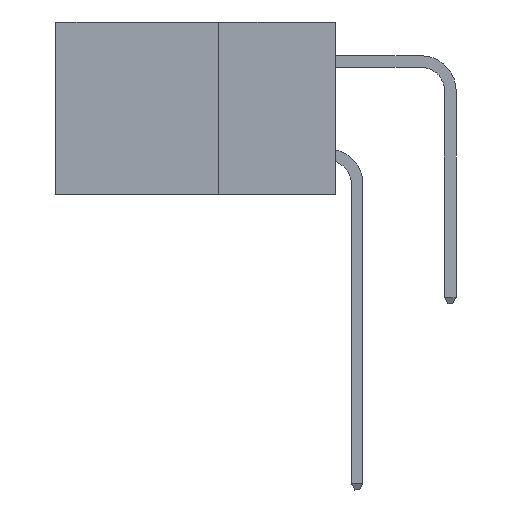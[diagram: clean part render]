
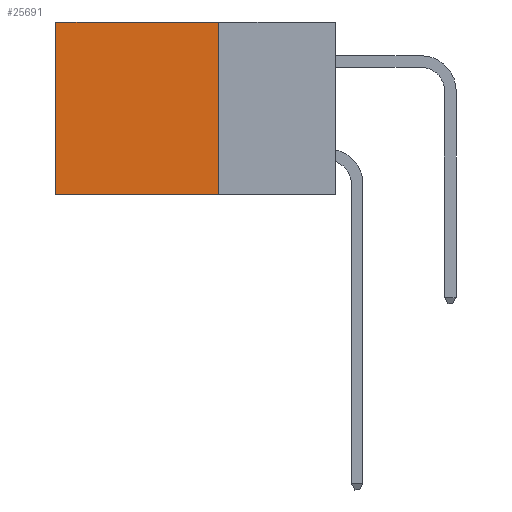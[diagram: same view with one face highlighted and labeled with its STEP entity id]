
A CAD part, left-side view. The second image highlights one B-rep face of the part: STEP entity #25691.
In plain terms, the highlighted planar face has unit normal (-1, 0, 0).
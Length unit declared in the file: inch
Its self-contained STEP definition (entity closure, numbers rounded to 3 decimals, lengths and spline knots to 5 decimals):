
#2548 = ORIENTED_EDGE ( 'NONE', *, *, #31524, .F. ) ;
#3533 = DIRECTION ( 'NONE',  ( 0., 0., -1. ) ) ;
#5704 = ORIENTED_EDGE ( 'NONE', *, *, #20865, .T. ) ;
#6212 = VECTOR ( 'NONE', #3533, 39.37008 ) ;
#8226 = EDGE_CURVE ( 'NONE', #35186, #17664, #32736, .T. ) ;
#8836 = DIRECTION ( 'NONE',  ( 0., 0., -1. ) ) ;
#9248 = FACE_OUTER_BOUND ( 'NONE', #13885, .T. ) ;
#9774 = DIRECTION ( 'NONE',  ( 0., 1., 0. ) ) ;
#9881 = VECTOR ( 'NONE', #24517, 39.37008 ) ;
#9988 = CARTESIAN_POINT ( 'NONE',  ( 0.2875, 0.25, -0.37 ) ) ;
#10068 = CARTESIAN_POINT ( 'NONE',  ( 0.2875, 0.25, 0. ) ) ;
#12613 = CARTESIAN_POINT ( 'NONE',  ( 0.2875, 0.6, 0. ) ) ;
#12982 = LINE ( 'NONE', #25811, #6212 ) ;
#13140 = LINE ( 'NONE', #9988, #15120 ) ;
#13885 = EDGE_LOOP ( 'NONE', ( #22132, #2548, #39092, #5704 ) ) ;
#14858 = LINE ( 'NONE', #27689, #9881 ) ;
#15120 = VECTOR ( 'NONE', #9774, 39.37008 ) ;
#16318 = CARTESIAN_POINT ( 'NONE',  ( 0.2875, 0.25, 0. ) ) ;
#17664 = VERTEX_POINT ( 'NONE', #25155 ) ;
#18876 = CARTESIAN_POINT ( 'NONE',  ( 0.2875, 0.6, -0.37 ) ) ;
#19999 = VECTOR ( 'NONE', #36100, 39.37008 ) ;
#20865 = EDGE_CURVE ( 'NONE', #35186, #25666, #14858, .T. ) ;
#22077 = PLANE ( 'NONE',  #39780 ) ;
#22132 = ORIENTED_EDGE ( 'NONE', *, *, #26334, .T. ) ;
#24517 = DIRECTION ( 'NONE',  ( 0., 1., 0. ) ) ;
#25155 = CARTESIAN_POINT ( 'NONE',  ( 0.2875, 0.25, -0.37 ) ) ;
#25666 = VERTEX_POINT ( 'NONE', #12613 ) ;
#25691 = ADVANCED_FACE ( 'NONE', ( #9248 ), #22077, .F. ) ;
#25811 = CARTESIAN_POINT ( 'NONE',  ( 0.2875, 0.6, 0. ) ) ;
#26334 = EDGE_CURVE ( 'NONE', #25666, #32419, #12982, .T. ) ;
#27689 = CARTESIAN_POINT ( 'NONE',  ( 0.2875, 0.25, 0. ) ) ;
#28607 = CARTESIAN_POINT ( 'NONE',  ( 0.2875, 0.25, 0. ) ) ;
#31349 = DIRECTION ( 'NONE',  ( 1., 0., 0. ) ) ;
#31524 = EDGE_CURVE ( 'NONE', #17664, #32419, #13140, .T. ) ;
#32419 = VERTEX_POINT ( 'NONE', #18876 ) ;
#32736 = LINE ( 'NONE', #16318, #19999 ) ;
#35186 = VERTEX_POINT ( 'NONE', #10068 ) ;
#36100 = DIRECTION ( 'NONE',  ( 0., 0., -1. ) ) ;
#39092 = ORIENTED_EDGE ( 'NONE', *, *, #8226, .F. ) ;
#39780 = AXIS2_PLACEMENT_3D ( 'NONE', #28607, #31349, #8836 ) ;
